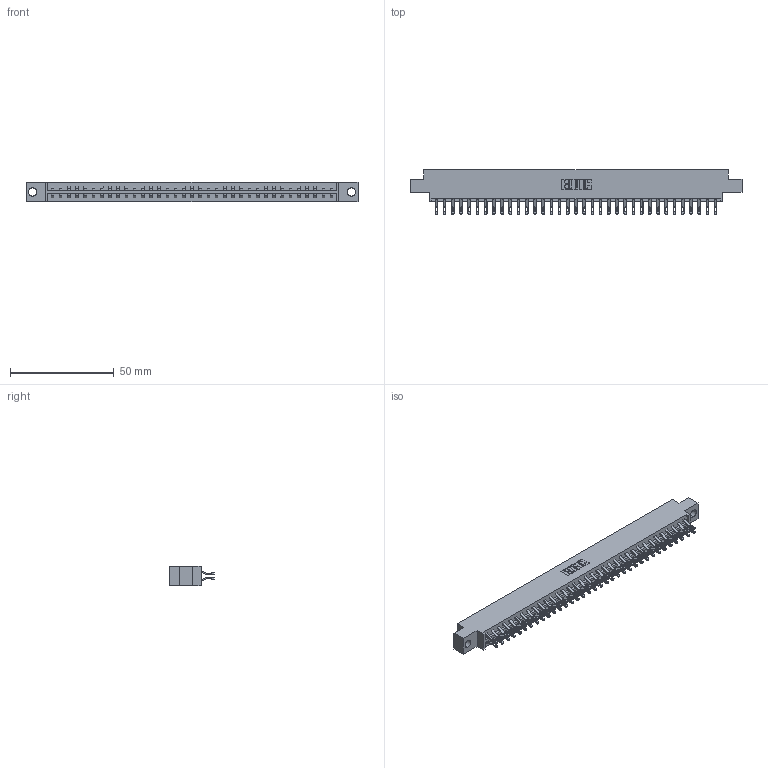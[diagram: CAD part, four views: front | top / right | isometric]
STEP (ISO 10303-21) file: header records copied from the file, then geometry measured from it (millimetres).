
FILE_DESCRIPTION (( 'STEP AP203' ), '1' );
FILE_NAME ('333-070-555-804.STEP', '2018-08-04T15:17:07', ( '' ), ( '' ), 'SwSTEP 2.0', 'SolidWorks 2016', '' );
FILE_SCHEMA (( 'CONFIG_CONTROL_DESIGN' ));
Length unit declared in the file: inch
Products named in the file (3): 333 Part_Offset - .156 Dia - TH; 345-292-001_555 Tail; 333-070-555-804
Assembly tree (71 placements, depth 2):
  333-070-555-804
    333 Part_Offset - .156 Dia - TH
    345-292-001_555 Tail  x70
Bounding box: 160.22 x 21.47 x 9.4 mm (x, y, z)
Volume: 16179.8 mm3; surface area: 19832.9 mm2
Topology: 71 solids, 71 shells, 4178 faces, 13133 edges, 8754 vertices
Faces by surface type: plane 2454, cylinder 1724
Entity records: 23883 total; most frequent: CARTESIAN_POINT 4004, ORIENTED_EDGE 3910, DIRECTION 3403, EDGE_CURVE 1955, LINE 1807, VECTOR 1807, VERTEX_POINT 1302, AXIS2_PLACEMENT_3D 798
